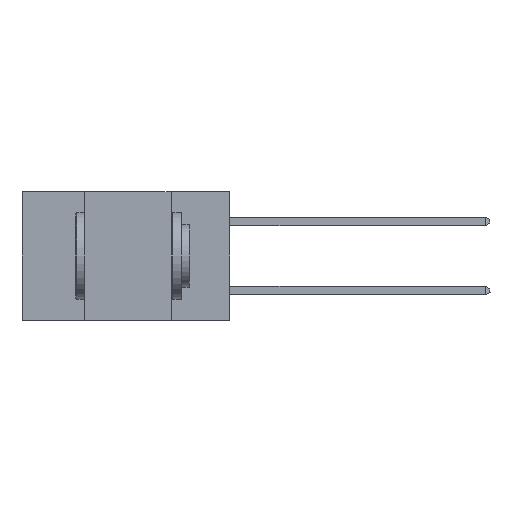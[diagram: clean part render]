
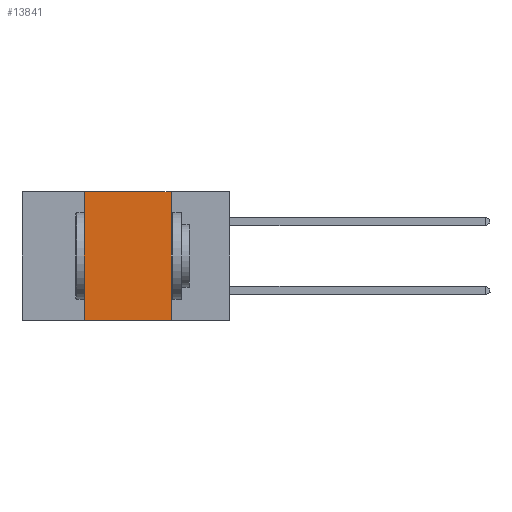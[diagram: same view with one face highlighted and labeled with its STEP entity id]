
A CAD part, left-side view. The second image highlights one B-rep face of the part: STEP entity #13841.
In plain terms, the highlighted planar face has unit normal (-1, 0, 0).
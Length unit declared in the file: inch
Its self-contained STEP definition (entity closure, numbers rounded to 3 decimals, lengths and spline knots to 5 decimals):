
#111 = EDGE_CURVE ( 'NONE', #15381, #20114, #11356, .T. ) ;
#1398 = DIRECTION ( 'NONE',  ( 0., 0., -1. ) ) ;
#1810 = EDGE_LOOP ( 'NONE', ( #6850, #4251, #9059, #15132 ) ) ;
#2219 = VECTOR ( 'NONE', #12026, 39.37008 ) ;
#4251 = ORIENTED_EDGE ( 'NONE', *, *, #13999, .F. ) ;
#6313 = VECTOR ( 'NONE', #21224, 39.37008 ) ;
#6850 = ORIENTED_EDGE ( 'NONE', *, *, #18755, .F. ) ;
#8566 = CARTESIAN_POINT ( 'NONE',  ( 0., 0.6, -0.37 ) ) ;
#9059 = ORIENTED_EDGE ( 'NONE', *, *, #12024, .F. ) ;
#9904 = VECTOR ( 'NONE', #19113, 39.37008 ) ;
#10794 = AXIS2_PLACEMENT_3D ( 'NONE', #15574, #17687, #1398 ) ;
#11356 = LINE ( 'NONE', #8566, #14749 ) ;
#11613 = LINE ( 'NONE', #21055, #2219 ) ;
#11881 = CARTESIAN_POINT ( 'NONE',  ( 0., 0.17, 0. ) ) ;
#11894 = CARTESIAN_POINT ( 'NONE',  ( 0., 0.42, 0. ) ) ;
#12024 = EDGE_CURVE ( 'NONE', #15381, #17374, #22667, .T. ) ;
#12026 = DIRECTION ( 'NONE',  ( 0., -1., 0. ) ) ;
#12377 = DIRECTION ( 'NONE',  ( 0., -1., 0. ) ) ;
#12597 = VERTEX_POINT ( 'NONE', #23351 ) ;
#13841 = ADVANCED_FACE ( 'NONE', ( #16623 ), #15889, .F. ) ;
#13999 = EDGE_CURVE ( 'NONE', #17374, #12597, #11613, .T. ) ;
#14749 = VECTOR ( 'NONE', #12377, 39.37008 ) ;
#15132 = ORIENTED_EDGE ( 'NONE', *, *, #111, .T. ) ;
#15381 = VERTEX_POINT ( 'NONE', #18414 ) ;
#15574 = CARTESIAN_POINT ( 'NONE',  ( 0., 0.6, 0. ) ) ;
#15889 = PLANE ( 'NONE',  #10794 ) ;
#16623 = FACE_OUTER_BOUND ( 'NONE', #1810, .T. ) ;
#16906 = CARTESIAN_POINT ( 'NONE',  ( 0., 0.42, 0. ) ) ;
#17374 = VERTEX_POINT ( 'NONE', #16906 ) ;
#17687 = DIRECTION ( 'NONE',  ( 1., 0., 0. ) ) ;
#17696 = LINE ( 'NONE', #11881, #6313 ) ;
#18414 = CARTESIAN_POINT ( 'NONE',  ( 0., 0.42, -0.37 ) ) ;
#18755 = EDGE_CURVE ( 'NONE', #12597, #20114, #17696, .T. ) ;
#19113 = DIRECTION ( 'NONE',  ( 0., 0., 1. ) ) ;
#19180 = CARTESIAN_POINT ( 'NONE',  ( 0., 0.17, -0.37 ) ) ;
#20114 = VERTEX_POINT ( 'NONE', #19180 ) ;
#21055 = CARTESIAN_POINT ( 'NONE',  ( 0., 0.6, 0. ) ) ;
#21224 = DIRECTION ( 'NONE',  ( 0., 0., -1. ) ) ;
#22667 = LINE ( 'NONE', #11894, #9904 ) ;
#23351 = CARTESIAN_POINT ( 'NONE',  ( 0., 0.17, 0. ) ) ;
